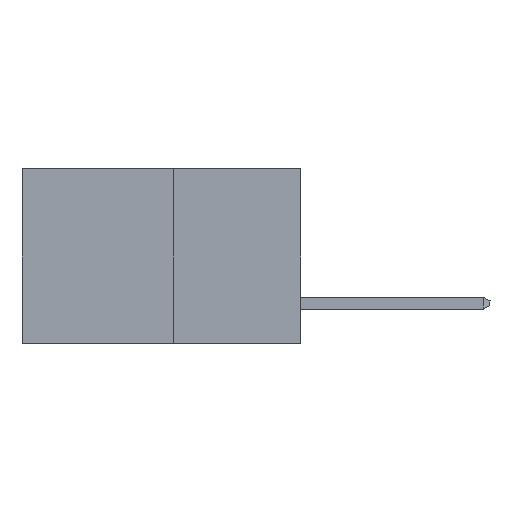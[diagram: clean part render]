
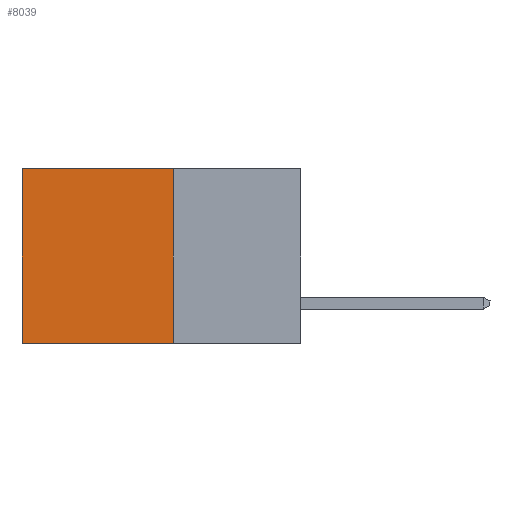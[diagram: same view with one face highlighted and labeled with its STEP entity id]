
A CAD part, left-side view. The second image highlights one B-rep face of the part: STEP entity #8039.
In plain terms, the highlighted planar face has unit normal (-1, 0, 0).
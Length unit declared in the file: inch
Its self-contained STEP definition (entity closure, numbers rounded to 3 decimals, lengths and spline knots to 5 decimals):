
#389 = VERTEX_POINT ( 'NONE', #3842 ) ;
#448 = VECTOR ( 'NONE', #4833, 39.37008 ) ;
#676 = CARTESIAN_POINT ( 'NONE',  ( 0.277, 0.27, 0. ) ) ;
#1163 = EDGE_CURVE ( 'NONE', #389, #6917, #7261, .T. ) ;
#2350 = VERTEX_POINT ( 'NONE', #7544 ) ;
#2516 = PLANE ( 'NONE',  #5492 ) ;
#2657 = DIRECTION ( 'NONE',  ( 0., 1., 0. ) ) ;
#3208 = DIRECTION ( 'NONE',  ( 0., 0., -1. ) ) ;
#3240 = EDGE_LOOP ( 'NONE', ( #8441, #5650, #3649, #6391 ) ) ;
#3402 = CARTESIAN_POINT ( 'NONE',  ( 0.277, 0.27, -0.37 ) ) ;
#3640 = DIRECTION ( 'NONE',  ( 0., 0., -1. ) ) ;
#3649 = ORIENTED_EDGE ( 'NONE', *, *, #8853, .F. ) ;
#3842 = CARTESIAN_POINT ( 'NONE',  ( 0.277, 0.59, 0. ) ) ;
#4112 = DIRECTION ( 'NONE',  ( 0., 0., -1. ) ) ;
#4116 = VERTEX_POINT ( 'NONE', #5328 ) ;
#4833 = DIRECTION ( 'NONE',  ( 0., 1., 0. ) ) ;
#4997 = VECTOR ( 'NONE', #4112, 39.37008 ) ;
#5240 = CARTESIAN_POINT ( 'NONE',  ( 0.277, 0.59, -0.37 ) ) ;
#5328 = CARTESIAN_POINT ( 'NONE',  ( 0.277, 0.27, -0.37 ) ) ;
#5492 = AXIS2_PLACEMENT_3D ( 'NONE', #7389, #7423, #3208 ) ;
#5650 = ORIENTED_EDGE ( 'NONE', *, *, #5717, .F. ) ;
#5717 = EDGE_CURVE ( 'NONE', #4116, #6917, #6210, .T. ) ;
#5999 = VECTOR ( 'NONE', #2657, 39.37008 ) ;
#6210 = LINE ( 'NONE', #8898, #5999 ) ;
#6391 = ORIENTED_EDGE ( 'NONE', *, *, #6639, .T. ) ;
#6639 = EDGE_CURVE ( 'NONE', #2350, #389, #7875, .T. ) ;
#6917 = VERTEX_POINT ( 'NONE', #5240 ) ;
#7181 = CARTESIAN_POINT ( 'NONE',  ( 0.277, 0.59, -0.37 ) ) ;
#7261 = LINE ( 'NONE', #7181, #8867 ) ;
#7389 = CARTESIAN_POINT ( 'NONE',  ( 0.277, 0.27, -0.37 ) ) ;
#7423 = DIRECTION ( 'NONE',  ( 1., 0., 0. ) ) ;
#7544 = CARTESIAN_POINT ( 'NONE',  ( 0.277, 0.27, 0. ) ) ;
#7875 = LINE ( 'NONE', #676, #448 ) ;
#8039 = ADVANCED_FACE ( 'NONE', ( #8377 ), #2516, .F. ) ;
#8377 = FACE_OUTER_BOUND ( 'NONE', #3240, .T. ) ;
#8441 = ORIENTED_EDGE ( 'NONE', *, *, #1163, .T. ) ;
#8696 = LINE ( 'NONE', #3402, #4997 ) ;
#8853 = EDGE_CURVE ( 'NONE', #2350, #4116, #8696, .T. ) ;
#8867 = VECTOR ( 'NONE', #3640, 39.37008 ) ;
#8898 = CARTESIAN_POINT ( 'NONE',  ( 0.277, 0.27, -0.37 ) ) ;
